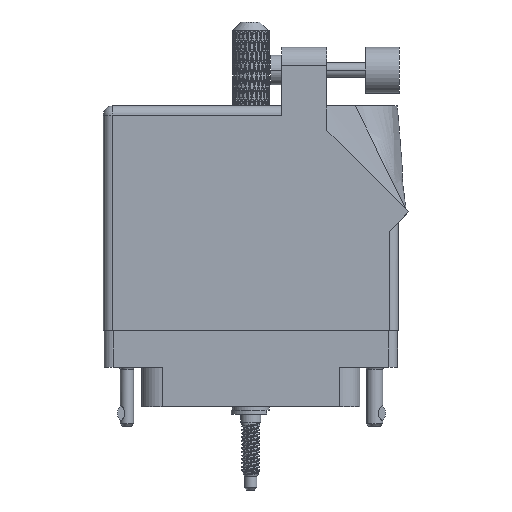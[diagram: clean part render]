
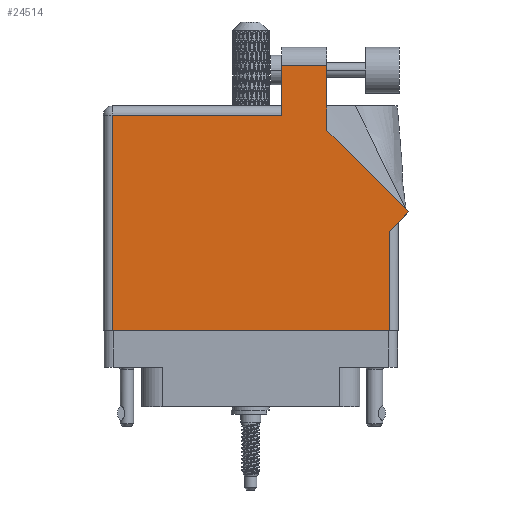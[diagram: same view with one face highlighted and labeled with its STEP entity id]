
A CAD part, front view. The second image highlights one B-rep face of the part: STEP entity #24514.
In plain terms, the highlighted face is planar.
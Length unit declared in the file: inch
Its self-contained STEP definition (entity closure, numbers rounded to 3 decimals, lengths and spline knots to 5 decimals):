
#4954 = LINE ( 'NONE', #38133, #86416 ) ;
#7070 = FACE_OUTER_BOUND ( 'NONE', #83771, .T. ) ;
#9143 = CARTESIAN_POINT ( 'NONE',  ( 0.519, 1.26442, 0.455 ) ) ;
#10528 = ORIENTED_EDGE ( 'NONE', *, *, #36171, .T. ) ;
#11316 = DIRECTION ( 'NONE',  ( -0.707, 0.707, 0. ) ) ;
#12504 = VECTOR ( 'NONE', #96869, 39.37008 ) ;
#13990 = ORIENTED_EDGE ( 'NONE', *, *, #33349, .T. ) ;
#14583 = DIRECTION ( 'NONE',  ( 0., 1., 0. ) ) ;
#14888 = VECTOR ( 'NONE', #65674, 39.37008 ) ;
#14920 = EDGE_CURVE ( 'NONE', #101503, #38858, #46226, .T. ) ;
#15212 = PLANE ( 'NONE',  #83084 ) ;
#16534 = DIRECTION ( 'NONE',  ( 0., -1., 0. ) ) ;
#21347 = VERTEX_POINT ( 'NONE', #91705 ) ;
#24514 = ADVANCED_FACE ( 'NONE', ( #7070 ), #15212, .F. ) ;
#25900 = ORIENTED_EDGE ( 'NONE', *, *, #99859, .T. ) ;
#26203 = ORIENTED_EDGE ( 'NONE', *, *, #30334, .T. ) ;
#29997 = DIRECTION ( 'NONE',  ( 0., -1., 0. ) ) ;
#30334 = EDGE_CURVE ( 'NONE', #61279, #113966, #4954, .T. ) ;
#32881 = VECTOR ( 'NONE', #58695, 39.37008 ) ;
#33349 = EDGE_CURVE ( 'NONE', #36616, #76415, #98328, .T. ) ;
#34489 = CARTESIAN_POINT ( 'NONE',  ( 1.07571, 0.70771, 0.455 ) ) ;
#36171 = EDGE_CURVE ( 'NONE', #49366, #36616, #93036, .T. ) ;
#36539 = CARTESIAN_POINT ( 'NONE',  ( -0.943, -0.1, 0.455 ) ) ;
#36616 = VERTEX_POINT ( 'NONE', #91741 ) ;
#36931 = CARTESIAN_POINT ( 'NONE',  ( 1.07571, 0.70771, 0.455 ) ) ;
#38133 = CARTESIAN_POINT ( 'NONE',  ( 0.212, 1.705, 0.455 ) ) ;
#38858 = VERTEX_POINT ( 'NONE', #9143 ) ;
#39065 = CARTESIAN_POINT ( 'NONE',  ( 0.519, 1.26442, 0.455 ) ) ;
#41985 = DIRECTION ( 'NONE',  ( 0., 0., -1. ) ) ;
#43847 = CARTESIAN_POINT ( 'NONE',  ( -0.943, -0.1, 0.455 ) ) ;
#45243 = ORIENTED_EDGE ( 'NONE', *, *, #61104, .T. ) ;
#46226 = LINE ( 'NONE', #36931, #89420 ) ;
#49354 = CARTESIAN_POINT ( 'NONE',  ( -1.005, -0.1, 0.455 ) ) ;
#49366 = VERTEX_POINT ( 'NONE', #36539 ) ;
#50593 = EDGE_CURVE ( 'NONE', #70685, #21347, #52594, .T. ) ;
#51533 = ORIENTED_EDGE ( 'NONE', *, *, #95867, .T. ) ;
#52325 = CARTESIAN_POINT ( 'NONE',  ( 0.943, 0.637, 0.455 ) ) ;
#52594 = LINE ( 'NONE', #88691, #12504 ) ;
#55004 = LINE ( 'NONE', #109738, #112597 ) ;
#57352 = ORIENTED_EDGE ( 'NONE', *, *, #14920, .T. ) ;
#58695 = DIRECTION ( 'NONE',  ( 0.707, 0.707, 0. ) ) ;
#61104 = EDGE_CURVE ( 'NONE', #21347, #49366, #88096, .T. ) ;
#61279 = VERTEX_POINT ( 'NONE', #93299 ) ;
#64542 = CARTESIAN_POINT ( 'NONE',  ( 1.005, 0.637, 0.455 ) ) ;
#65674 = DIRECTION ( 'NONE',  ( 1., 0., 0. ) ) ;
#67624 = CARTESIAN_POINT ( 'NONE',  ( -1.005, 1.43, 0.455 ) ) ;
#68326 = CARTESIAN_POINT ( 'NONE',  ( 0.212, 1.705, 0.455 ) ) ;
#70109 = VECTOR ( 'NONE', #14583, 39.37008 ) ;
#70685 = VERTEX_POINT ( 'NONE', #92626 ) ;
#76415 = VERTEX_POINT ( 'NONE', #110404 ) ;
#77520 = DIRECTION ( 'NONE',  ( -1., 0., 0. ) ) ;
#78594 = ORIENTED_EDGE ( 'NONE', *, *, #99474, .T. ) ;
#83084 = AXIS2_PLACEMENT_3D ( 'NONE', #67624, #41985, #77520 ) ;
#83771 = EDGE_LOOP ( 'NONE', ( #78594, #26203, #51533, #84042, #45243, #10528, #13990, #25900, #57352 ) ) ;
#84042 = ORIENTED_EDGE ( 'NONE', *, *, #50593, .T. ) ;
#86416 = VECTOR ( 'NONE', #100990, 39.37008 ) ;
#88096 = LINE ( 'NONE', #43847, #90725 ) ;
#88434 = DIRECTION ( 'NONE',  ( 0., 1., 0. ) ) ;
#88691 = CARTESIAN_POINT ( 'NONE',  ( -1.005, 1.368, 0.455 ) ) ;
#89420 = VECTOR ( 'NONE', #11316, 39.37008 ) ;
#90725 = VECTOR ( 'NONE', #16534, 39.37008 ) ;
#91705 = CARTESIAN_POINT ( 'NONE',  ( -0.943, 1.368, 0.455 ) ) ;
#91741 = CARTESIAN_POINT ( 'NONE',  ( 0.943, -0.1, 0.455 ) ) ;
#92626 = CARTESIAN_POINT ( 'NONE',  ( 0.212, 1.368, 0.455 ) ) ;
#93036 = LINE ( 'NONE', #49354, #14888 ) ;
#93299 = CARTESIAN_POINT ( 'NONE',  ( 0.519, 1.705, 0.455 ) ) ;
#95867 = EDGE_CURVE ( 'NONE', #113966, #70685, #55004, .T. ) ;
#96869 = DIRECTION ( 'NONE',  ( -1., 0., 0. ) ) ;
#98328 = LINE ( 'NONE', #52325, #113133 ) ;
#99474 = EDGE_CURVE ( 'NONE', #38858, #61279, #101912, .T. ) ;
#99859 = EDGE_CURVE ( 'NONE', #76415, #101503, #107608, .T. ) ;
#100990 = DIRECTION ( 'NONE',  ( -1., 0., 0. ) ) ;
#101503 = VERTEX_POINT ( 'NONE', #34489 ) ;
#101912 = LINE ( 'NONE', #39065, #70109 ) ;
#107608 = LINE ( 'NONE', #64542, #32881 ) ;
#109738 = CARTESIAN_POINT ( 'NONE',  ( 0.212, 1.43, 0.455 ) ) ;
#110404 = CARTESIAN_POINT ( 'NONE',  ( 0.943, 0.575, 0.455 ) ) ;
#112597 = VECTOR ( 'NONE', #29997, 39.37008 ) ;
#113133 = VECTOR ( 'NONE', #88434, 39.37008 ) ;
#113966 = VERTEX_POINT ( 'NONE', #68326 ) ;
